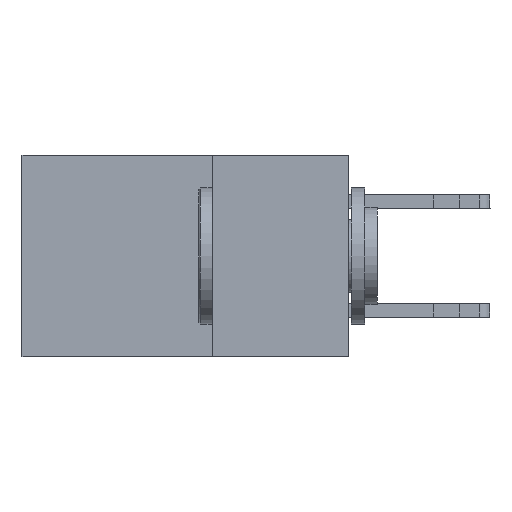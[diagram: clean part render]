
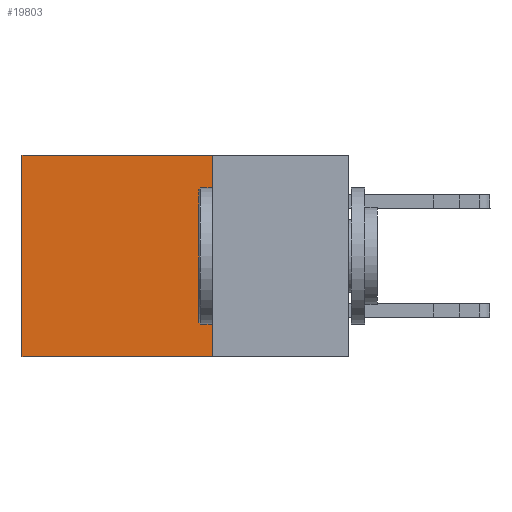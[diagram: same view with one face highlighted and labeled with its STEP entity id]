
A CAD part, left-side view. The second image highlights one B-rep face of the part: STEP entity #19803.
In plain terms, the highlighted planar face has unit normal (-1, 0, 0).
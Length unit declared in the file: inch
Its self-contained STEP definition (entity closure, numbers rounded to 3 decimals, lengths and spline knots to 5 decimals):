
#10 = CARTESIAN_POINT ( 'NONE',  ( 0.2615, 0.25, 0. ) ) ;
#294 = VERTEX_POINT ( 'NONE', #11826 ) ;
#569 = LINE ( 'NONE', #13631, #4286 ) ;
#735 = LINE ( 'NONE', #3630, #5024 ) ;
#1845 = LINE ( 'NONE', #6115, #16386 ) ;
#2230 = VERTEX_POINT ( 'NONE', #7695 ) ;
#3630 = CARTESIAN_POINT ( 'NONE',  ( 0.2615, 0.25, -0.37 ) ) ;
#3876 = ORIENTED_EDGE ( 'NONE', *, *, #18481, .T. ) ;
#4286 = VECTOR ( 'NONE', #9957, 39.37008 ) ;
#4682 = ORIENTED_EDGE ( 'NONE', *, *, #16940, .F. ) ;
#5024 = VECTOR ( 'NONE', #18195, 39.37008 ) ;
#5074 = VERTEX_POINT ( 'NONE', #10990 ) ;
#5893 = EDGE_LOOP ( 'NONE', ( #3876, #17119, #4682, #11070 ) ) ;
#6115 = CARTESIAN_POINT ( 'NONE',  ( 0.2615, 0.6, -0.37 ) ) ;
#6362 = DIRECTION ( 'NONE',  ( 1., 0., 0. ) ) ;
#7405 = EDGE_CURVE ( 'NONE', #15380, #294, #9175, .T. ) ;
#7695 = CARTESIAN_POINT ( 'NONE',  ( 0.2615, 0.25, -0.37 ) ) ;
#8612 = EDGE_CURVE ( 'NONE', #2230, #5074, #569, .T. ) ;
#8669 = CARTESIAN_POINT ( 'NONE',  ( 0.2615, 0.25, 0. ) ) ;
#9175 = LINE ( 'NONE', #8669, #23094 ) ;
#9436 = AXIS2_PLACEMENT_3D ( 'NONE', #9917, #6362, #19084 ) ;
#9917 = CARTESIAN_POINT ( 'NONE',  ( 0.2615, 0.25, -0.37 ) ) ;
#9957 = DIRECTION ( 'NONE',  ( 0., 1., 0. ) ) ;
#10499 = DIRECTION ( 'NONE',  ( 0., 1., 0. ) ) ;
#10990 = CARTESIAN_POINT ( 'NONE',  ( 0.2615, 0.6, -0.37 ) ) ;
#11070 = ORIENTED_EDGE ( 'NONE', *, *, #7405, .T. ) ;
#11826 = CARTESIAN_POINT ( 'NONE',  ( 0.2615, 0.6, 0. ) ) ;
#13631 = CARTESIAN_POINT ( 'NONE',  ( 0.2615, 0.25, -0.37 ) ) ;
#15380 = VERTEX_POINT ( 'NONE', #10 ) ;
#16386 = VECTOR ( 'NONE', #22401, 39.37008 ) ;
#16940 = EDGE_CURVE ( 'NONE', #15380, #2230, #735, .T. ) ;
#17119 = ORIENTED_EDGE ( 'NONE', *, *, #8612, .F. ) ;
#17283 = PLANE ( 'NONE',  #9436 ) ;
#17476 = FACE_OUTER_BOUND ( 'NONE', #5893, .T. ) ;
#18195 = DIRECTION ( 'NONE',  ( 0., 0., -1. ) ) ;
#18481 = EDGE_CURVE ( 'NONE', #294, #5074, #1845, .T. ) ;
#19084 = DIRECTION ( 'NONE',  ( 0., 0., -1. ) ) ;
#19803 = ADVANCED_FACE ( 'NONE', ( #17476 ), #17283, .F. ) ;
#22401 = DIRECTION ( 'NONE',  ( 0., 0., -1. ) ) ;
#23094 = VECTOR ( 'NONE', #10499, 39.37008 ) ;
